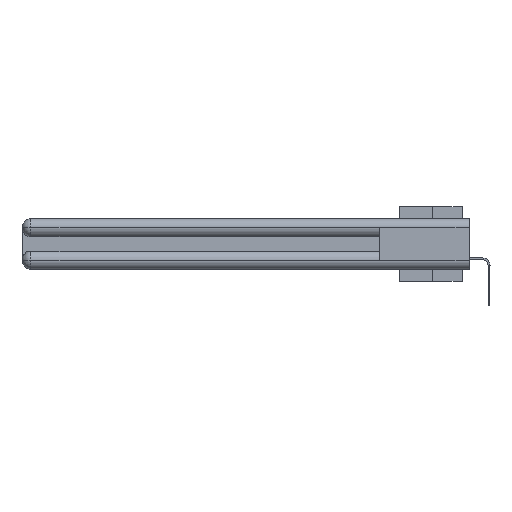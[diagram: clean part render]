
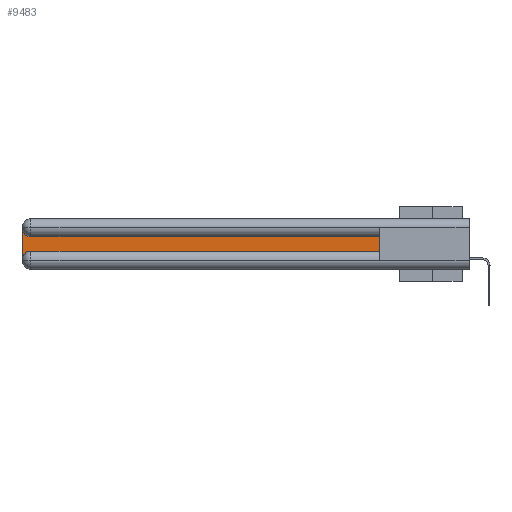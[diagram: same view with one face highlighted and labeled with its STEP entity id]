
A CAD part, left-side view. The second image highlights one B-rep face of the part: STEP entity #9483.
In plain terms, the highlighted planar face has unit normal (-1, 0, 0).
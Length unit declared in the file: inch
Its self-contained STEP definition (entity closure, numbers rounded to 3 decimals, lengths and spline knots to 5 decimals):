
#1521 = EDGE_CURVE ( 'NONE', #14862, #21750, #15457, .T. ) ;
#1537 = VECTOR ( 'NONE', #4592, 39.37008 ) ;
#1749 = PLANE ( 'NONE',  #28599 ) ;
#2826 = EDGE_CURVE ( 'NONE', #23874, #14862, #15404, .T. ) ;
#3283 = VECTOR ( 'NONE', #23527, 39.37008 ) ;
#3394 = VERTEX_POINT ( 'NONE', #20568 ) ;
#3887 = CARTESIAN_POINT ( 'NONE',  ( 0.075, 0.6, -0.1225 ) ) ;
#4592 = DIRECTION ( 'NONE',  ( 0., -1., 0. ) ) ;
#5407 = DIRECTION ( 'NONE',  ( 0., 0., -1. ) ) ;
#5415 = ORIENTED_EDGE ( 'NONE', *, *, #2826, .T. ) ;
#7063 = VERTEX_POINT ( 'NONE', #11387 ) ;
#8050 = CIRCLE ( 'NONE', #8328, 0.06 ) ;
#8184 = DIRECTION ( 'NONE',  ( 0., 0., 1. ) ) ;
#8203 = EDGE_CURVE ( 'NONE', #21750, #3394, #11521, .T. ) ;
#8328 = AXIS2_PLACEMENT_3D ( 'NONE', #24372, #17098, #9871 ) ;
#8612 = EDGE_CURVE ( 'NONE', #3394, #20465, #8819, .T. ) ;
#8819 = LINE ( 'NONE', #14895, #17187 ) ;
#9298 = CARTESIAN_POINT ( 'NONE',  ( 0.075, 3., -0.1225 ) ) ;
#9483 = ADVANCED_FACE ( 'NONE', ( #19762 ), #1749, .F. ) ;
#9499 = DIRECTION ( 'NONE',  ( 0., 0., -1. ) ) ;
#9784 = DIRECTION ( 'NONE',  ( 1., 0., 0. ) ) ;
#9871 = DIRECTION ( 'NONE',  ( 0., 0., -1. ) ) ;
#11387 = CARTESIAN_POINT ( 'NONE',  ( 0.075, 2.94, -0.2175 ) ) ;
#11521 = CIRCLE ( 'NONE', #15419, 0.06 ) ;
#14477 = DIRECTION ( 'NONE',  ( 0., 0., -1. ) ) ;
#14517 = ORIENTED_EDGE ( 'NONE', *, *, #21133, .T. ) ;
#14862 = VERTEX_POINT ( 'NONE', #3887 ) ;
#14895 = CARTESIAN_POINT ( 'NONE',  ( 0.075, 3., -0.2175 ) ) ;
#14935 = ORIENTED_EDGE ( 'NONE', *, *, #8203, .T. ) ;
#15404 = LINE ( 'NONE', #29916, #30881 ) ;
#15419 = AXIS2_PLACEMENT_3D ( 'NONE', #19232, #9784, #14477 ) ;
#15457 = LINE ( 'NONE', #28178, #3283 ) ;
#16016 = CARTESIAN_POINT ( 'NONE',  ( 0.075, 0.6, -0.2175 ) ) ;
#16577 = ORIENTED_EDGE ( 'NONE', *, *, #19481, .T. ) ;
#17098 = DIRECTION ( 'NONE',  ( 1., 0., 0. ) ) ;
#17187 = VECTOR ( 'NONE', #5407, 39.37008 ) ;
#19232 = CARTESIAN_POINT ( 'NONE',  ( 0.075, 2.94, -0.0625 ) ) ;
#19481 = EDGE_CURVE ( 'NONE', #20465, #7063, #8050, .T. ) ;
#19762 = FACE_OUTER_BOUND ( 'NONE', #28094, .T. ) ;
#20465 = VERTEX_POINT ( 'NONE', #28715 ) ;
#20568 = CARTESIAN_POINT ( 'NONE',  ( 0.075, 3., -0.0625 ) ) ;
#21072 = ORIENTED_EDGE ( 'NONE', *, *, #1521, .T. ) ;
#21133 = EDGE_CURVE ( 'NONE', #7063, #23874, #22801, .T. ) ;
#21750 = VERTEX_POINT ( 'NONE', #29377 ) ;
#22801 = LINE ( 'NONE', #26668, #1537 ) ;
#23527 = DIRECTION ( 'NONE',  ( 0., 1., 0. ) ) ;
#23707 = DIRECTION ( 'NONE',  ( 1., 0., 0. ) ) ;
#23874 = VERTEX_POINT ( 'NONE', #16016 ) ;
#24372 = CARTESIAN_POINT ( 'NONE',  ( 0.075, 2.94, -0.2775 ) ) ;
#26668 = CARTESIAN_POINT ( 'NONE',  ( 0.075, 0.6, -0.2175 ) ) ;
#28094 = EDGE_LOOP ( 'NONE', ( #21072, #14935, #31015, #16577, #14517, #5415 ) ) ;
#28178 = CARTESIAN_POINT ( 'NONE',  ( 0.075, 0.6, -0.1225 ) ) ;
#28599 = AXIS2_PLACEMENT_3D ( 'NONE', #9298, #23707, #9499 ) ;
#28715 = CARTESIAN_POINT ( 'NONE',  ( 0.075, 3., -0.2775 ) ) ;
#29377 = CARTESIAN_POINT ( 'NONE',  ( 0.075, 2.94, -0.1225 ) ) ;
#29916 = CARTESIAN_POINT ( 'NONE',  ( 0.075, 0.6, -0.2175 ) ) ;
#30881 = VECTOR ( 'NONE', #8184, 39.37008 ) ;
#31015 = ORIENTED_EDGE ( 'NONE', *, *, #8612, .T. ) ;
